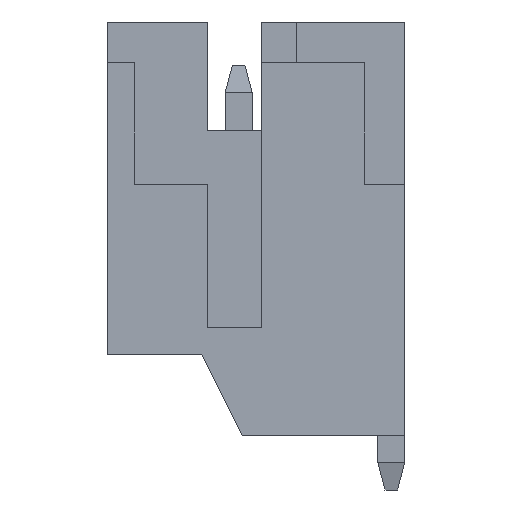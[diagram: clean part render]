
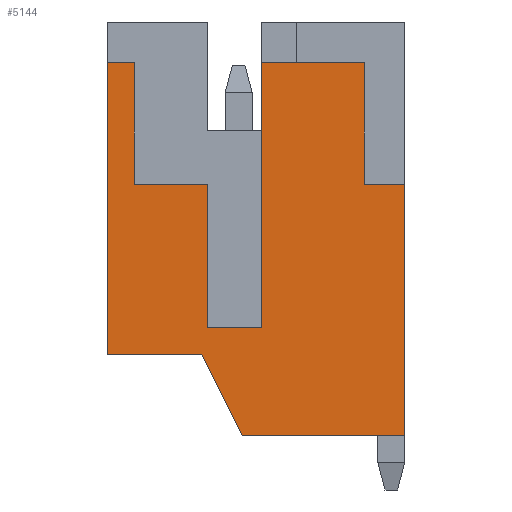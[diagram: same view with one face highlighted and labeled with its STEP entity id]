
A CAD part, left-side view. The second image highlights one B-rep face of the part: STEP entity #5144.
In plain terms, the highlighted planar face has unit normal (-1, 0, 0).
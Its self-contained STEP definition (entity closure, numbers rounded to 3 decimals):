
#213 = VERTEX_POINT ( 'NONE', #281 ) ;
#230 = VECTOR ( 'NONE', #2373, 1000. ) ;
#281 = CARTESIAN_POINT ( 'NONE',  ( -3., -2.32, 5.4 ) ) ;
#340 = VECTOR ( 'NONE', #5089, 1000. ) ;
#368 = DIRECTION ( 'NONE',  ( 0., -1., 0. ) ) ;
#580 = CARTESIAN_POINT ( 'NONE',  ( -3., -0.42, 6.15 ) ) ;
#626 = DIRECTION ( 'NONE',  ( -1., 0., 0. ) ) ;
#638 = VECTOR ( 'NONE', #2095, 1000. ) ;
#762 = VERTEX_POINT ( 'NONE', #2226 ) ;
#811 = VERTEX_POINT ( 'NONE', #2183 ) ;
#975 = CARTESIAN_POINT ( 'NONE',  ( -3., -0.07, -1.5 ) ) ;
#1148 = VERTEX_POINT ( 'NONE', #3565 ) ;
#1268 = VERTEX_POINT ( 'NONE', #2669 ) ;
#1297 = CARTESIAN_POINT ( 'NONE',  ( -3., 0.68, 0. ) ) ;
#1301 = LINE ( 'NONE', #2243, #6047 ) ;
#1379 = LINE ( 'NONE', #6389, #230 ) ;
#1398 = CARTESIAN_POINT ( 'NONE',  ( -3., -2.32, 3.15 ) ) ;
#1478 = DIRECTION ( 'NONE',  ( 0., -0.447, -0.894 ) ) ;
#1485 = LINE ( 'NONE', #1398, #4753 ) ;
#1570 = VECTOR ( 'NONE', #1478, 1000. ) ;
#1644 = CARTESIAN_POINT ( 'NONE',  ( -3., 0.58, 0.5 ) ) ;
#1667 = DIRECTION ( 'NONE',  ( 0., 0., -1. ) ) ;
#1697 = ORIENTED_EDGE ( 'NONE', *, *, #3534, .T. ) ;
#1847 = VERTEX_POINT ( 'NONE', #2331 ) ;
#1912 = CARTESIAN_POINT ( 'NONE',  ( -3., 2.43, 0. ) ) ;
#1953 = DIRECTION ( 'NONE',  ( 0., -1., 0. ) ) ;
#1964 = VECTOR ( 'NONE', #4258, 1000. ) ;
#2095 = DIRECTION ( 'NONE',  ( 0., 0., -1. ) ) ;
#2156 = VERTEX_POINT ( 'NONE', #5181 ) ;
#2183 = CARTESIAN_POINT ( 'NONE',  ( -3., 1.93, 5.4 ) ) ;
#2191 = LINE ( 'NONE', #5756, #1964 ) ;
#2217 = EDGE_CURVE ( 'NONE', #811, #1847, #2430, .T. ) ;
#2226 = CARTESIAN_POINT ( 'NONE',  ( -3., -2.32, 3.15 ) ) ;
#2243 = CARTESIAN_POINT ( 'NONE',  ( -3., 1.93, 3.15 ) ) ;
#2252 = DIRECTION ( 'NONE',  ( 0., 1., 0. ) ) ;
#2331 = CARTESIAN_POINT ( 'NONE',  ( -3., 2.43, 5.4 ) ) ;
#2373 = DIRECTION ( 'NONE',  ( 0., 0., 1. ) ) ;
#2411 = VECTOR ( 'NONE', #4355, 1000. ) ;
#2428 = VERTEX_POINT ( 'NONE', #6232 ) ;
#2430 = LINE ( 'NONE', #4223, #3985 ) ;
#2449 = AXIS2_PLACEMENT_3D ( 'NONE', #6024, #626, #3055 ) ;
#2473 = VECTOR ( 'NONE', #3377, 1000. ) ;
#2527 = EDGE_CURVE ( 'NONE', #3786, #2156, #5608, .T. ) ;
#2572 = LINE ( 'NONE', #2728, #4666 ) ;
#2598 = EDGE_LOOP ( 'NONE', ( #2960, #6266, #1697, #2862, #5287, #4194, #3864, #2796, #5516, #4946, #5333, #5967, #5130, #5655 ) ) ;
#2661 = CARTESIAN_POINT ( 'NONE',  ( -3., -3.07, -1.5 ) ) ;
#2669 = CARTESIAN_POINT ( 'NONE',  ( -3., 0.58, 3.15 ) ) ;
#2728 = CARTESIAN_POINT ( 'NONE',  ( -3., 2.43, 6.15 ) ) ;
#2792 = CARTESIAN_POINT ( 'NONE',  ( -3., -3.07, -1.5 ) ) ;
#2796 = ORIENTED_EDGE ( 'NONE', *, *, #4381, .T. ) ;
#2862 = ORIENTED_EDGE ( 'NONE', *, *, #2527, .T. ) ;
#2960 = ORIENTED_EDGE ( 'NONE', *, *, #2217, .T. ) ;
#3020 = VERTEX_POINT ( 'NONE', #1644 ) ;
#3055 = DIRECTION ( 'NONE',  ( 0., -1., 0. ) ) ;
#3124 = CARTESIAN_POINT ( 'NONE',  ( -3., -3.07, 3.15 ) ) ;
#3188 = CARTESIAN_POINT ( 'NONE',  ( -3., -2.32, 3.15 ) ) ;
#3290 = EDGE_CURVE ( 'NONE', #762, #3379, #1485, .T. ) ;
#3349 = FACE_OUTER_BOUND ( 'NONE', #2598, .T. ) ;
#3377 = DIRECTION ( 'NONE',  ( 0., -1., 0. ) ) ;
#3379 = VERTEX_POINT ( 'NONE', #3124 ) ;
#3534 = EDGE_CURVE ( 'NONE', #5928, #3786, #5832, .T. ) ;
#3565 = CARTESIAN_POINT ( 'NONE',  ( -3., -0.42, 5.4 ) ) ;
#3737 = VECTOR ( 'NONE', #1953, 1000. ) ;
#3742 = EDGE_CURVE ( 'NONE', #1268, #3020, #2191, .T. ) ;
#3786 = VERTEX_POINT ( 'NONE', #1297 ) ;
#3827 = DIRECTION ( 'NONE',  ( 0., 0., 1. ) ) ;
#3864 = ORIENTED_EDGE ( 'NONE', *, *, #3290, .F. ) ;
#3971 = LINE ( 'NONE', #5400, #5140 ) ;
#3985 = VECTOR ( 'NONE', #2252, 1000. ) ;
#4007 = EDGE_CURVE ( 'NONE', #213, #1148, #3971, .T. ) ;
#4194 = ORIENTED_EDGE ( 'NONE', *, *, #5588, .T. ) ;
#4223 = CARTESIAN_POINT ( 'NONE',  ( -3., -3.07, 5.4 ) ) ;
#4258 = DIRECTION ( 'NONE',  ( 0., 0., -1. ) ) ;
#4325 = VERTEX_POINT ( 'NONE', #2661 ) ;
#4332 = EDGE_CURVE ( 'NONE', #1847, #5928, #2572, .T. ) ;
#4345 = CARTESIAN_POINT ( 'NONE',  ( -3., -0.42, 0.5 ) ) ;
#4355 = DIRECTION ( 'NONE',  ( 0., 0., 1. ) ) ;
#4381 = EDGE_CURVE ( 'NONE', #762, #213, #5677, .T. ) ;
#4422 = VECTOR ( 'NONE', #5684, 1000. ) ;
#4443 = DIRECTION ( 'NONE',  ( 0., 1., 0. ) ) ;
#4666 = VECTOR ( 'NONE', #1667, 1000. ) ;
#4753 = VECTOR ( 'NONE', #368, 1000. ) ;
#4845 = EDGE_CURVE ( 'NONE', #1148, #2428, #5366, .T. ) ;
#4946 = ORIENTED_EDGE ( 'NONE', *, *, #4845, .T. ) ;
#4967 = EDGE_CURVE ( 'NONE', #5793, #1268, #5741, .T. ) ;
#5041 = LINE ( 'NONE', #4345, #2473 ) ;
#5087 = EDGE_CURVE ( 'NONE', #2156, #4325, #5521, .T. ) ;
#5089 = DIRECTION ( 'NONE',  ( 0., -1., 0. ) ) ;
#5130 = ORIENTED_EDGE ( 'NONE', *, *, #4967, .F. ) ;
#5140 = VECTOR ( 'NONE', #4443, 1000. ) ;
#5144 = ADVANCED_FACE ( 'NONE', ( #3349 ), #6000, .T. ) ;
#5181 = CARTESIAN_POINT ( 'NONE',  ( -3., -0.07, -1.5 ) ) ;
#5287 = ORIENTED_EDGE ( 'NONE', *, *, #5087, .T. ) ;
#5333 = ORIENTED_EDGE ( 'NONE', *, *, #5937, .F. ) ;
#5366 = LINE ( 'NONE', #580, #638 ) ;
#5400 = CARTESIAN_POINT ( 'NONE',  ( -3., -3.07, 5.4 ) ) ;
#5516 = ORIENTED_EDGE ( 'NONE', *, *, #4007, .T. ) ;
#5521 = LINE ( 'NONE', #2792, #3737 ) ;
#5563 = CARTESIAN_POINT ( 'NONE',  ( -3., 2.43, 0. ) ) ;
#5588 = EDGE_CURVE ( 'NONE', #4325, #3379, #1379, .T. ) ;
#5608 = LINE ( 'NONE', #975, #1570 ) ;
#5655 = ORIENTED_EDGE ( 'NONE', *, *, #5784, .T. ) ;
#5665 = CARTESIAN_POINT ( 'NONE',  ( -3., -0.42, 3.15 ) ) ;
#5677 = LINE ( 'NONE', #3188, #2411 ) ;
#5684 = DIRECTION ( 'NONE',  ( 0., -1., 0. ) ) ;
#5741 = LINE ( 'NONE', #5665, #4422 ) ;
#5756 = CARTESIAN_POINT ( 'NONE',  ( -3., 0.58, 3.15 ) ) ;
#5784 = EDGE_CURVE ( 'NONE', #5793, #811, #1301, .T. ) ;
#5793 = VERTEX_POINT ( 'NONE', #6282 ) ;
#5832 = LINE ( 'NONE', #5563, #340 ) ;
#5928 = VERTEX_POINT ( 'NONE', #1912 ) ;
#5937 = EDGE_CURVE ( 'NONE', #3020, #2428, #5041, .T. ) ;
#5967 = ORIENTED_EDGE ( 'NONE', *, *, #3742, .F. ) ;
#6000 = PLANE ( 'NONE',  #2449 ) ;
#6024 = CARTESIAN_POINT ( 'NONE',  ( -3., 0., 0. ) ) ;
#6047 = VECTOR ( 'NONE', #3827, 1000. ) ;
#6232 = CARTESIAN_POINT ( 'NONE',  ( -3., -0.42, 0.5 ) ) ;
#6266 = ORIENTED_EDGE ( 'NONE', *, *, #4332, .T. ) ;
#6282 = CARTESIAN_POINT ( 'NONE',  ( -3., 1.93, 3.15 ) ) ;
#6389 = CARTESIAN_POINT ( 'NONE',  ( -3., -3.07, 6.15 ) ) ;
